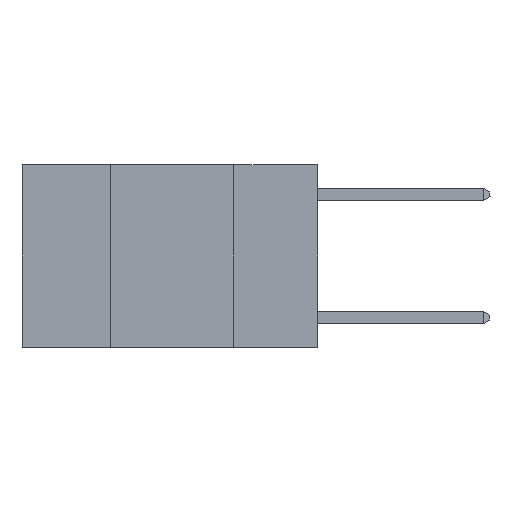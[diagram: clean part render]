
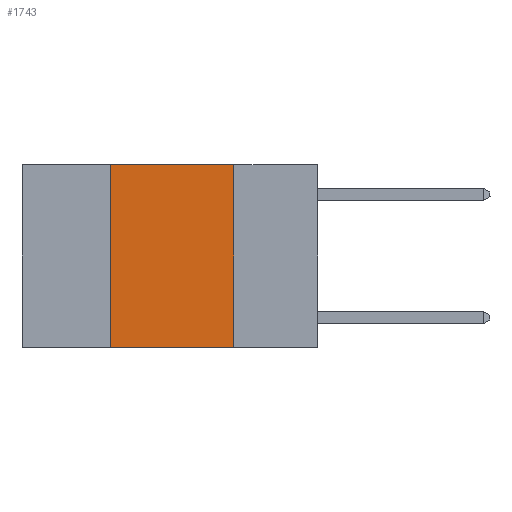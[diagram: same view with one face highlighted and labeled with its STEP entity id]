
A CAD part, left-side view. The second image highlights one B-rep face of the part: STEP entity #1743.
In plain terms, the highlighted planar face has unit normal (-1, 0, 0).
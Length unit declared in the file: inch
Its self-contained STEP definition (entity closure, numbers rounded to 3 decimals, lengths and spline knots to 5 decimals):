
#213 = EDGE_CURVE ( 'NONE', #4436, #3896, #1080, .T. ) ;
#371 = CARTESIAN_POINT ( 'NONE',  ( 0., 0.17, 0. ) ) ;
#865 = VERTEX_POINT ( 'NONE', #6774 ) ;
#879 = VECTOR ( 'NONE', #1129, 39.37008 ) ;
#1027 = VERTEX_POINT ( 'NONE', #6180 ) ;
#1071 = LINE ( 'NONE', #6924, #3984 ) ;
#1080 = LINE ( 'NONE', #3553, #879 ) ;
#1129 = DIRECTION ( 'NONE',  ( 0., 0., 1. ) ) ;
#1634 = ORIENTED_EDGE ( 'NONE', *, *, #2084, .F. ) ;
#1743 = ADVANCED_FACE ( 'NONE', ( #2502 ), #3742, .F. ) ;
#2084 = EDGE_CURVE ( 'NONE', #3896, #1027, #2193, .T. ) ;
#2175 = ORIENTED_EDGE ( 'NONE', *, *, #213, .F. ) ;
#2193 = LINE ( 'NONE', #4833, #3574 ) ;
#2343 = CARTESIAN_POINT ( 'NONE',  ( 0., 0.42, -0.37 ) ) ;
#2502 = FACE_OUTER_BOUND ( 'NONE', #8113, .T. ) ;
#3553 = CARTESIAN_POINT ( 'NONE',  ( 0., 0.42, 0. ) ) ;
#3574 = VECTOR ( 'NONE', #6139, 39.37008 ) ;
#3742 = PLANE ( 'NONE',  #4773 ) ;
#3766 = DIRECTION ( 'NONE',  ( 0., 0., -1. ) ) ;
#3786 = DIRECTION ( 'NONE',  ( 1., 0., 0. ) ) ;
#3896 = VERTEX_POINT ( 'NONE', #7299 ) ;
#3984 = VECTOR ( 'NONE', #6179, 39.37008 ) ;
#4430 = LINE ( 'NONE', #371, #5883 ) ;
#4436 = VERTEX_POINT ( 'NONE', #2343 ) ;
#4773 = AXIS2_PLACEMENT_3D ( 'NONE', #6268, #3786, #7540 ) ;
#4833 = CARTESIAN_POINT ( 'NONE',  ( 0., 0.6, 0. ) ) ;
#5883 = VECTOR ( 'NONE', #3766, 39.37008 ) ;
#6139 = DIRECTION ( 'NONE',  ( 0., -1., 0. ) ) ;
#6161 = EDGE_CURVE ( 'NONE', #1027, #865, #4430, .T. ) ;
#6179 = DIRECTION ( 'NONE',  ( 0., -1., 0. ) ) ;
#6180 = CARTESIAN_POINT ( 'NONE',  ( 0., 0.17, 0. ) ) ;
#6268 = CARTESIAN_POINT ( 'NONE',  ( 0., 0.6, 0. ) ) ;
#6299 = ORIENTED_EDGE ( 'NONE', *, *, #7184, .T. ) ;
#6774 = CARTESIAN_POINT ( 'NONE',  ( 0., 0.17, -0.37 ) ) ;
#6924 = CARTESIAN_POINT ( 'NONE',  ( 0., 0.6, -0.37 ) ) ;
#7184 = EDGE_CURVE ( 'NONE', #4436, #865, #1071, .T. ) ;
#7299 = CARTESIAN_POINT ( 'NONE',  ( 0., 0.42, 0. ) ) ;
#7368 = ORIENTED_EDGE ( 'NONE', *, *, #6161, .F. ) ;
#7540 = DIRECTION ( 'NONE',  ( 0., 0., -1. ) ) ;
#8113 = EDGE_LOOP ( 'NONE', ( #7368, #1634, #2175, #6299 ) ) ;
